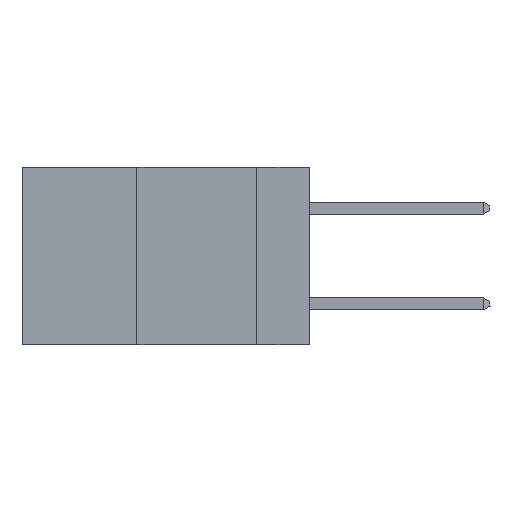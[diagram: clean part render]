
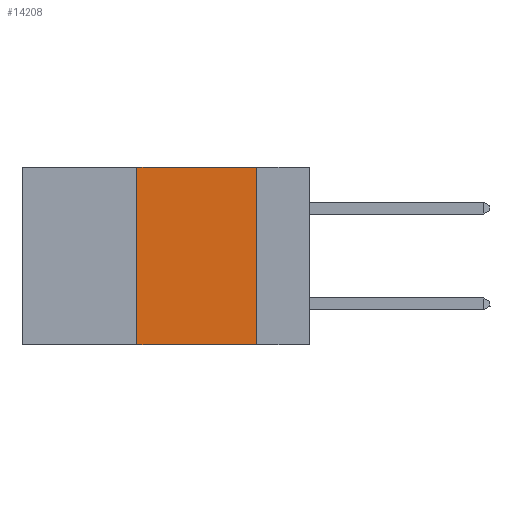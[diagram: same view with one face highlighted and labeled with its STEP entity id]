
A CAD part, left-side view. The second image highlights one B-rep face of the part: STEP entity #14208.
In plain terms, the highlighted planar face has unit normal (-1, 0, 0).
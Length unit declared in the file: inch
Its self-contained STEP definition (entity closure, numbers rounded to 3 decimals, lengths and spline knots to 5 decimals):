
#503 = LINE ( 'NONE', #8290, #11873 ) ;
#554 = EDGE_CURVE ( 'NONE', #5904, #9402, #1850, .T. ) ;
#1262 = CARTESIAN_POINT ( 'NONE',  ( 0., 0.6, -0.37 ) ) ;
#1850 = LINE ( 'NONE', #1262, #8340 ) ;
#2621 = CARTESIAN_POINT ( 'NONE',  ( 0., 0.6, 0. ) ) ;
#2787 = DIRECTION ( 'NONE',  ( 0., -1., 0. ) ) ;
#3962 = DIRECTION ( 'NONE',  ( 1., 0., 0. ) ) ;
#4389 = LINE ( 'NONE', #14651, #8148 ) ;
#4633 = CARTESIAN_POINT ( 'NONE',  ( 0., 0.11, -0.37 ) ) ;
#5029 = ORIENTED_EDGE ( 'NONE', *, *, #13546, .F. ) ;
#5268 = ORIENTED_EDGE ( 'NONE', *, *, #554, .T. ) ;
#5474 = CARTESIAN_POINT ( 'NONE',  ( 0., 0.36, -0.37 ) ) ;
#5798 = FACE_OUTER_BOUND ( 'NONE', #13881, .T. ) ;
#5904 = VERTEX_POINT ( 'NONE', #5474 ) ;
#6036 = VERTEX_POINT ( 'NONE', #15917 ) ;
#6715 = PLANE ( 'NONE',  #16788 ) ;
#7109 = CARTESIAN_POINT ( 'NONE',  ( 0., 0.36, 0. ) ) ;
#8148 = VECTOR ( 'NONE', #2787, 39.37008 ) ;
#8290 = CARTESIAN_POINT ( 'NONE',  ( 0., 0.11, 0. ) ) ;
#8340 = VECTOR ( 'NONE', #9279, 39.37008 ) ;
#8533 = LINE ( 'NONE', #15450, #13603 ) ;
#9279 = DIRECTION ( 'NONE',  ( 0., -1., 0. ) ) ;
#9402 = VERTEX_POINT ( 'NONE', #4633 ) ;
#9695 = ORIENTED_EDGE ( 'NONE', *, *, #15438, .F. ) ;
#10106 = DIRECTION ( 'NONE',  ( 0., 0., 1. ) ) ;
#10913 = DIRECTION ( 'NONE',  ( 0., 0., -1. ) ) ;
#11618 = EDGE_CURVE ( 'NONE', #5904, #15170, #8533, .T. ) ;
#11873 = VECTOR ( 'NONE', #10913, 39.37008 ) ;
#13546 = EDGE_CURVE ( 'NONE', #15170, #6036, #4389, .T. ) ;
#13603 = VECTOR ( 'NONE', #10106, 39.37008 ) ;
#13881 = EDGE_LOOP ( 'NONE', ( #9695, #5029, #16211, #5268 ) ) ;
#14208 = ADVANCED_FACE ( 'NONE', ( #5798 ), #6715, .F. ) ;
#14651 = CARTESIAN_POINT ( 'NONE',  ( 0., 0.6, 0. ) ) ;
#14715 = DIRECTION ( 'NONE',  ( 0., 0., -1. ) ) ;
#15170 = VERTEX_POINT ( 'NONE', #7109 ) ;
#15438 = EDGE_CURVE ( 'NONE', #6036, #9402, #503, .T. ) ;
#15450 = CARTESIAN_POINT ( 'NONE',  ( 0., 0.36, 0. ) ) ;
#15917 = CARTESIAN_POINT ( 'NONE',  ( 0., 0.11, 0. ) ) ;
#16211 = ORIENTED_EDGE ( 'NONE', *, *, #11618, .F. ) ;
#16788 = AXIS2_PLACEMENT_3D ( 'NONE', #2621, #3962, #14715 ) ;
